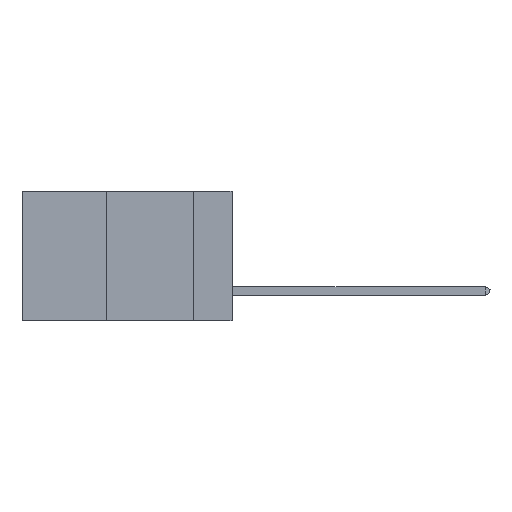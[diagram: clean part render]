
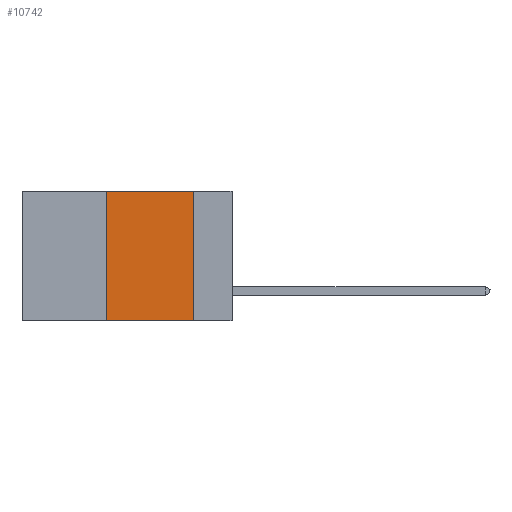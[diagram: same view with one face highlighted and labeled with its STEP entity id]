
A CAD part, left-side view. The second image highlights one B-rep face of the part: STEP entity #10742.
In plain terms, the highlighted planar face has unit normal (-1, 0, 0).
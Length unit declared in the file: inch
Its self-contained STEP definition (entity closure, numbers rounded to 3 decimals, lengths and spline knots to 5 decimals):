
#1559 = PLANE ( 'NONE',  #24409 ) ;
#1659 = ORIENTED_EDGE ( 'NONE', *, *, #23291, .F. ) ;
#1716 = VERTEX_POINT ( 'NONE', #19693 ) ;
#1784 = CARTESIAN_POINT ( 'NONE',  ( 0., 0.11, 0. ) ) ;
#1875 = EDGE_CURVE ( 'NONE', #1716, #8963, #25389, .T. ) ;
#1879 = LINE ( 'NONE', #22107, #15406 ) ;
#2313 = CARTESIAN_POINT ( 'NONE',  ( 0., 0.11, -0.37 ) ) ;
#3477 = DIRECTION ( 'NONE',  ( 0., 0., -1. ) ) ;
#4090 = DIRECTION ( 'NONE',  ( 0., -1., 0. ) ) ;
#6814 = EDGE_CURVE ( 'NONE', #21492, #8963, #16331, .T. ) ;
#6871 = CARTESIAN_POINT ( 'NONE',  ( 0., 0.36, 0. ) ) ;
#7120 = ORIENTED_EDGE ( 'NONE', *, *, #1875, .T. ) ;
#7303 = CARTESIAN_POINT ( 'NONE',  ( 0., 0.6, 0. ) ) ;
#8963 = VERTEX_POINT ( 'NONE', #2313 ) ;
#9322 = DIRECTION ( 'NONE',  ( 0., -1., 0. ) ) ;
#9788 = DIRECTION ( 'NONE',  ( 0., 0., -1. ) ) ;
#9803 = ORIENTED_EDGE ( 'NONE', *, *, #6814, .F. ) ;
#10058 = DIRECTION ( 'NONE',  ( 0., 0., 1. ) ) ;
#10742 = ADVANCED_FACE ( 'NONE', ( #24282 ), #1559, .F. ) ;
#10968 = VECTOR ( 'NONE', #9788, 39.37008 ) ;
#11242 = VECTOR ( 'NONE', #4090, 39.37008 ) ;
#11546 = EDGE_LOOP ( 'NONE', ( #9803, #22242, #1659, #7120 ) ) ;
#15023 = VECTOR ( 'NONE', #9322, 39.37008 ) ;
#15406 = VECTOR ( 'NONE', #10058, 39.37008 ) ;
#15551 = CARTESIAN_POINT ( 'NONE',  ( 0., 0.6, 0. ) ) ;
#16331 = LINE ( 'NONE', #1784, #10968 ) ;
#18320 = EDGE_CURVE ( 'NONE', #25293, #21492, #25707, .T. ) ;
#19608 = CARTESIAN_POINT ( 'NONE',  ( 0., 0.11, 0. ) ) ;
#19693 = CARTESIAN_POINT ( 'NONE',  ( 0., 0.36, -0.37 ) ) ;
#21492 = VERTEX_POINT ( 'NONE', #19608 ) ;
#22107 = CARTESIAN_POINT ( 'NONE',  ( 0., 0.36, 0. ) ) ;
#22242 = ORIENTED_EDGE ( 'NONE', *, *, #18320, .F. ) ;
#22282 = CARTESIAN_POINT ( 'NONE',  ( 0., 0.6, -0.37 ) ) ;
#23291 = EDGE_CURVE ( 'NONE', #1716, #25293, #1879, .T. ) ;
#23460 = DIRECTION ( 'NONE',  ( 1., 0., 0. ) ) ;
#24282 = FACE_OUTER_BOUND ( 'NONE', #11546, .T. ) ;
#24409 = AXIS2_PLACEMENT_3D ( 'NONE', #15551, #23460, #3477 ) ;
#25293 = VERTEX_POINT ( 'NONE', #6871 ) ;
#25389 = LINE ( 'NONE', #22282, #11242 ) ;
#25707 = LINE ( 'NONE', #7303, #15023 ) ;
